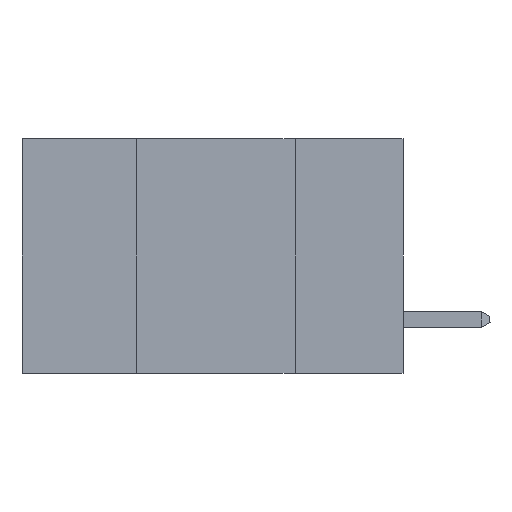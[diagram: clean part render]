
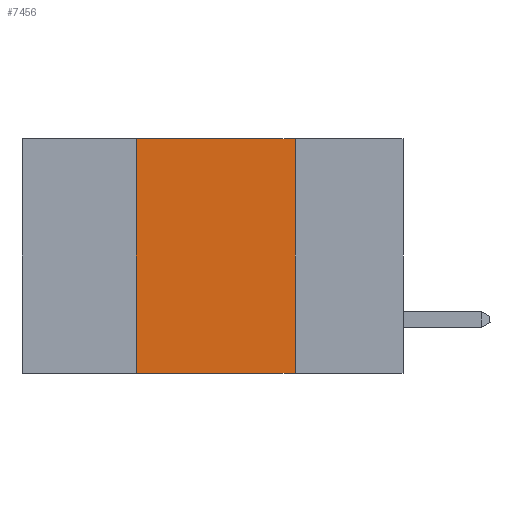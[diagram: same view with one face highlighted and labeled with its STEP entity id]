
A CAD part, left-side view. The second image highlights one B-rep face of the part: STEP entity #7456.
In plain terms, the highlighted planar face has unit normal (-1, 0, 0).
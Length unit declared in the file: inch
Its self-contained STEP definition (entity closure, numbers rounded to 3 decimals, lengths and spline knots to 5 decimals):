
#2556 = VERTEX_POINT ( 'NONE', #5989 ) ;
#2697 = CARTESIAN_POINT ( 'NONE',  ( 0., 0.17, -0.37 ) ) ;
#3936 = LINE ( 'NONE', #13918, #11771 ) ;
#5156 = DIRECTION ( 'NONE',  ( 0., -1., 0. ) ) ;
#5989 = CARTESIAN_POINT ( 'NONE',  ( 0., 0.42, -0.37 ) ) ;
#6253 = CARTESIAN_POINT ( 'NONE',  ( 0., 0.42, 0. ) ) ;
#7130 = CARTESIAN_POINT ( 'NONE',  ( 0., 0.17, 0. ) ) ;
#7456 = ADVANCED_FACE ( 'NONE', ( #10824 ), #17262, .F. ) ;
#7647 = EDGE_CURVE ( 'NONE', #2556, #17077, #16996, .T. ) ;
#8050 = VECTOR ( 'NONE', #15721, 39.37008 ) ;
#8252 = CARTESIAN_POINT ( 'NONE',  ( 0., 0.42, 0. ) ) ;
#8530 = EDGE_LOOP ( 'NONE', ( #8838, #10467, #15534, #17018 ) ) ;
#8594 = DIRECTION ( 'NONE',  ( 0., 0., -1. ) ) ;
#8838 = ORIENTED_EDGE ( 'NONE', *, *, #11894, .F. ) ;
#9326 = VECTOR ( 'NONE', #5156, 39.37008 ) ;
#10467 = ORIENTED_EDGE ( 'NONE', *, *, #15012, .F. ) ;
#10824 = FACE_OUTER_BOUND ( 'NONE', #8530, .T. ) ;
#11651 = LINE ( 'NONE', #6253, #8050 ) ;
#11728 = CARTESIAN_POINT ( 'NONE',  ( 0., 0.6, -0.37 ) ) ;
#11771 = VECTOR ( 'NONE', #8594, 39.37008 ) ;
#11824 = DIRECTION ( 'NONE',  ( 1., 0., 0. ) ) ;
#11894 = EDGE_CURVE ( 'NONE', #14222, #17077, #3936, .T. ) ;
#12917 = LINE ( 'NONE', #15917, #9326 ) ;
#13439 = DIRECTION ( 'NONE',  ( 0., -1., 0. ) ) ;
#13918 = CARTESIAN_POINT ( 'NONE',  ( 0., 0.17, 0. ) ) ;
#14185 = VERTEX_POINT ( 'NONE', #8252 ) ;
#14192 = AXIS2_PLACEMENT_3D ( 'NONE', #17201, #11824, #14551 ) ;
#14222 = VERTEX_POINT ( 'NONE', #7130 ) ;
#14267 = VECTOR ( 'NONE', #13439, 39.37008 ) ;
#14551 = DIRECTION ( 'NONE',  ( 0., 0., -1. ) ) ;
#15012 = EDGE_CURVE ( 'NONE', #14185, #14222, #12917, .T. ) ;
#15496 = EDGE_CURVE ( 'NONE', #2556, #14185, #11651, .T. ) ;
#15534 = ORIENTED_EDGE ( 'NONE', *, *, #15496, .F. ) ;
#15721 = DIRECTION ( 'NONE',  ( 0., 0., 1. ) ) ;
#15917 = CARTESIAN_POINT ( 'NONE',  ( 0., 0.6, 0. ) ) ;
#16996 = LINE ( 'NONE', #11728, #14267 ) ;
#17018 = ORIENTED_EDGE ( 'NONE', *, *, #7647, .T. ) ;
#17077 = VERTEX_POINT ( 'NONE', #2697 ) ;
#17201 = CARTESIAN_POINT ( 'NONE',  ( 0., 0.6, 0. ) ) ;
#17262 = PLANE ( 'NONE',  #14192 ) ;
